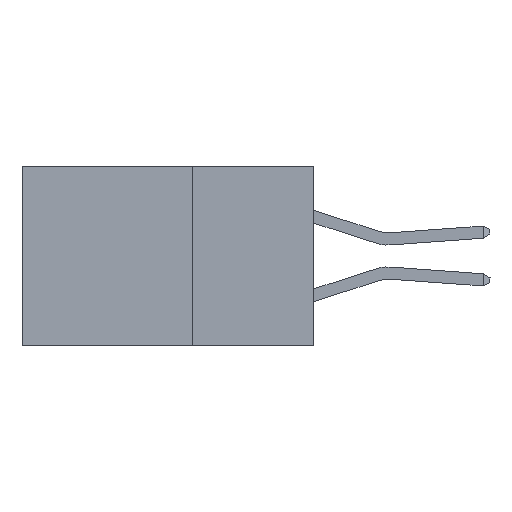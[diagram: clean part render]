
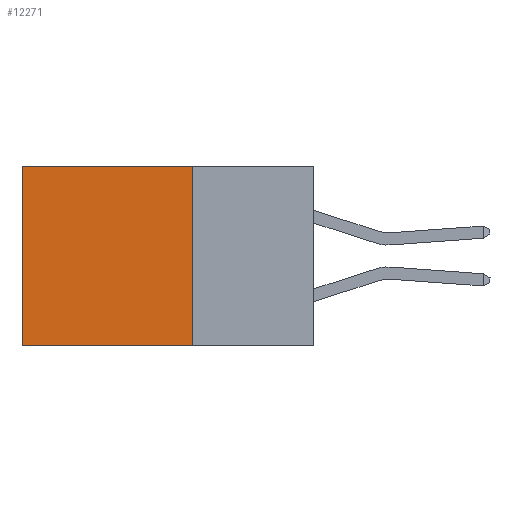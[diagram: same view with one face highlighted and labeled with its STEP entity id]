
A CAD part, left-side view. The second image highlights one B-rep face of the part: STEP entity #12271.
In plain terms, the highlighted planar face has unit normal (-1, 0, 0).
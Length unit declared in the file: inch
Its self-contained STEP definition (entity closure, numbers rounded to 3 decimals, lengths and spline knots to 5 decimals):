
#505 = VECTOR ( 'NONE', #4908, 39.37008 ) ;
#680 = LINE ( 'NONE', #10070, #505 ) ;
#751 = DIRECTION ( 'NONE',  ( 0., 0., -1. ) ) ;
#1530 = ORIENTED_EDGE ( 'NONE', *, *, #4774, .F. ) ;
#1653 = ORIENTED_EDGE ( 'NONE', *, *, #1932, .F. ) ;
#1820 = EDGE_CURVE ( 'NONE', #6240, #11925, #8988, .T. ) ;
#1932 = EDGE_CURVE ( 'NONE', #12820, #11925, #4724, .T. ) ;
#2000 = VECTOR ( 'NONE', #9980, 39.37008 ) ;
#2306 = PLANE ( 'NONE',  #3372 ) ;
#3208 = CARTESIAN_POINT ( 'NONE',  ( 0.2875, 0.25, 0. ) ) ;
#3372 = AXIS2_PLACEMENT_3D ( 'NONE', #3208, #9611, #7436 ) ;
#3765 = CARTESIAN_POINT ( 'NONE',  ( 0.2875, 0.25, 0. ) ) ;
#4021 = CARTESIAN_POINT ( 'NONE',  ( 0.2875, 0.6, 0. ) ) ;
#4724 = LINE ( 'NONE', #7153, #11135 ) ;
#4774 = EDGE_CURVE ( 'NONE', #8584, #12820, #7968, .T. ) ;
#4908 = DIRECTION ( 'NONE',  ( 0., 1., 0. ) ) ;
#5725 = CARTESIAN_POINT ( 'NONE',  ( 0.2875, 0.6, 0. ) ) ;
#6240 = VERTEX_POINT ( 'NONE', #4021 ) ;
#6597 = CARTESIAN_POINT ( 'NONE',  ( 0.2875, 0.25, 0. ) ) ;
#6617 = EDGE_LOOP ( 'NONE', ( #9599, #1653, #1530, #8348 ) ) ;
#7153 = CARTESIAN_POINT ( 'NONE',  ( 0.2875, 0.25, -0.37 ) ) ;
#7436 = DIRECTION ( 'NONE',  ( 0., 0., -1. ) ) ;
#7968 = LINE ( 'NONE', #3765, #13330 ) ;
#8221 = DIRECTION ( 'NONE',  ( 0., 1., 0. ) ) ;
#8348 = ORIENTED_EDGE ( 'NONE', *, *, #12128, .T. ) ;
#8584 = VERTEX_POINT ( 'NONE', #6597 ) ;
#8988 = LINE ( 'NONE', #5725, #2000 ) ;
#9599 = ORIENTED_EDGE ( 'NONE', *, *, #1820, .T. ) ;
#9611 = DIRECTION ( 'NONE',  ( 1., 0., 0. ) ) ;
#9626 = CARTESIAN_POINT ( 'NONE',  ( 0.2875, 0.25, -0.37 ) ) ;
#9980 = DIRECTION ( 'NONE',  ( 0., 0., -1. ) ) ;
#10070 = CARTESIAN_POINT ( 'NONE',  ( 0.2875, 0.25, 0. ) ) ;
#10615 = FACE_OUTER_BOUND ( 'NONE', #6617, .T. ) ;
#10939 = CARTESIAN_POINT ( 'NONE',  ( 0.2875, 0.6, -0.37 ) ) ;
#11135 = VECTOR ( 'NONE', #8221, 39.37008 ) ;
#11925 = VERTEX_POINT ( 'NONE', #10939 ) ;
#12128 = EDGE_CURVE ( 'NONE', #8584, #6240, #680, .T. ) ;
#12271 = ADVANCED_FACE ( 'NONE', ( #10615 ), #2306, .F. ) ;
#12820 = VERTEX_POINT ( 'NONE', #9626 ) ;
#13330 = VECTOR ( 'NONE', #751, 39.37008 ) ;
